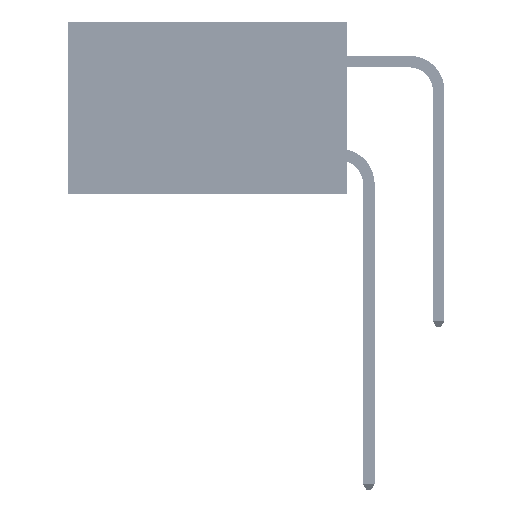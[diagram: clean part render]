
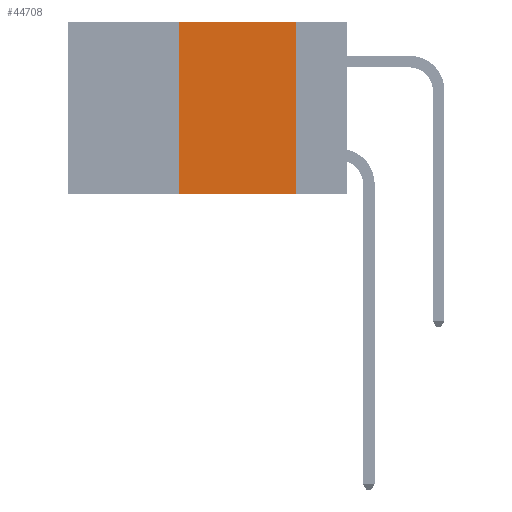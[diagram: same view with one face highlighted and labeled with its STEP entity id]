
A CAD part, left-side view. The second image highlights one B-rep face of the part: STEP entity #44708.
In plain terms, the highlighted planar face has unit normal (-1, 0, 0).
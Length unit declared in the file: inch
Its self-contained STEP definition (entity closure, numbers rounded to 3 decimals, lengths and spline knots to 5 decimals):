
#3739 = VECTOR ( 'NONE', #4859, 39.37008 ) ;
#4233 = EDGE_CURVE ( 'NONE', #7871, #29847, #48809, .T. ) ;
#4759 = CARTESIAN_POINT ( 'NONE',  ( 0., 0.6, -0.37 ) ) ;
#4859 = DIRECTION ( 'NONE',  ( 0., -1., 0. ) ) ;
#4905 = LINE ( 'NONE', #27532, #3739 ) ;
#7871 = VERTEX_POINT ( 'NONE', #28114 ) ;
#9263 = DIRECTION ( 'NONE',  ( 0., 0., 1. ) ) ;
#9342 = EDGE_LOOP ( 'NONE', ( #27780, #38318, #12551, #36016 ) ) ;
#12551 = ORIENTED_EDGE ( 'NONE', *, *, #20324, .F. ) ;
#12920 = VECTOR ( 'NONE', #19448, 39.37008 ) ;
#17029 = LINE ( 'NONE', #4759, #12920 ) ;
#17680 = VERTEX_POINT ( 'NONE', #35858 ) ;
#17681 = CARTESIAN_POINT ( 'NONE',  ( 0., 0.11, -0.37 ) ) ;
#19448 = DIRECTION ( 'NONE',  ( 0., -1., 0. ) ) ;
#20324 = EDGE_CURVE ( 'NONE', #25090, #17680, #25002, .T. ) ;
#24132 = CARTESIAN_POINT ( 'NONE',  ( 0., 0.36, 0. ) ) ;
#25002 = LINE ( 'NONE', #24132, #45787 ) ;
#25090 = VERTEX_POINT ( 'NONE', #37946 ) ;
#26145 = DIRECTION ( 'NONE',  ( 0., 0., -1. ) ) ;
#27532 = CARTESIAN_POINT ( 'NONE',  ( 0., 0.6, 0. ) ) ;
#27780 = ORIENTED_EDGE ( 'NONE', *, *, #4233, .F. ) ;
#28114 = CARTESIAN_POINT ( 'NONE',  ( 0., 0.11, 0. ) ) ;
#29271 = AXIS2_PLACEMENT_3D ( 'NONE', #37810, #45593, #34007 ) ;
#29847 = VERTEX_POINT ( 'NONE', #17681 ) ;
#30913 = EDGE_CURVE ( 'NONE', #25090, #29847, #17029, .T. ) ;
#32636 = FACE_OUTER_BOUND ( 'NONE', #9342, .T. ) ;
#33798 = EDGE_CURVE ( 'NONE', #17680, #7871, #4905, .T. ) ;
#34007 = DIRECTION ( 'NONE',  ( 0., 0., -1. ) ) ;
#34184 = PLANE ( 'NONE',  #29271 ) ;
#35858 = CARTESIAN_POINT ( 'NONE',  ( 0., 0.36, 0. ) ) ;
#36016 = ORIENTED_EDGE ( 'NONE', *, *, #30913, .T. ) ;
#37565 = VECTOR ( 'NONE', #26145, 39.37008 ) ;
#37810 = CARTESIAN_POINT ( 'NONE',  ( 0., 0.6, 0. ) ) ;
#37946 = CARTESIAN_POINT ( 'NONE',  ( 0., 0.36, -0.37 ) ) ;
#38318 = ORIENTED_EDGE ( 'NONE', *, *, #33798, .F. ) ;
#44708 = ADVANCED_FACE ( 'NONE', ( #32636 ), #34184, .F. ) ;
#45593 = DIRECTION ( 'NONE',  ( 1., 0., 0. ) ) ;
#45787 = VECTOR ( 'NONE', #9263, 39.37008 ) ;
#48809 = LINE ( 'NONE', #48855, #37565 ) ;
#48855 = CARTESIAN_POINT ( 'NONE',  ( 0., 0.11, 0. ) ) ;
